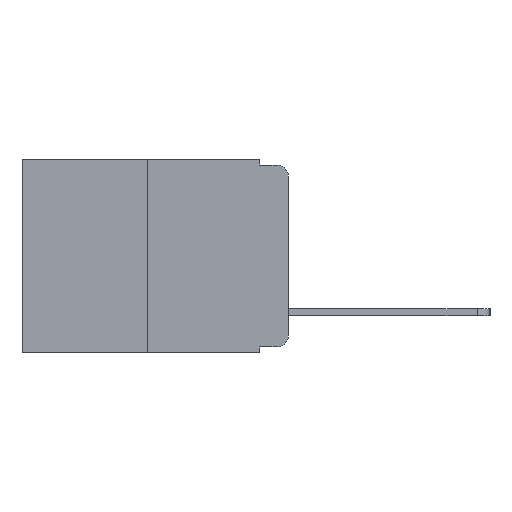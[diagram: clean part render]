
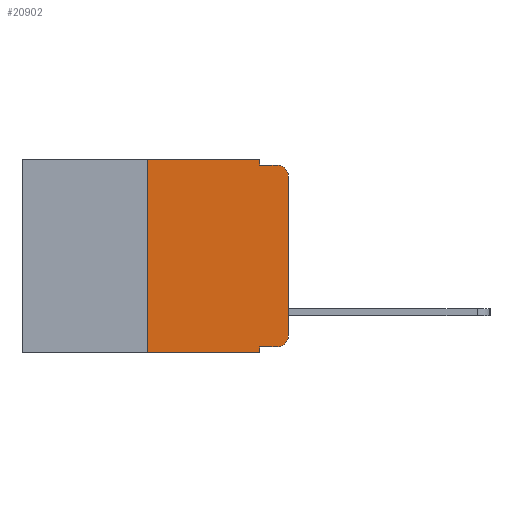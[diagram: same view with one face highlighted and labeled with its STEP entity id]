
A CAD part, left-side view. The second image highlights one B-rep face of the part: STEP entity #20902.
In plain terms, the highlighted planar face has unit normal (-1, 0, 0).
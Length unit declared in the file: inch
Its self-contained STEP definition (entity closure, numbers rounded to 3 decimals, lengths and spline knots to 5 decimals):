
#699 = LINE ( 'NONE', #13658, #19922 ) ;
#744 = VERTEX_POINT ( 'NONE', #4660 ) ;
#796 = VERTEX_POINT ( 'NONE', #8427 ) ;
#1297 = CARTESIAN_POINT ( 'NONE',  ( 0., 0.051, 0. ) ) ;
#1508 = EDGE_CURVE ( 'NONE', #4152, #19162, #22091, .T. ) ;
#1558 = VECTOR ( 'NONE', #15631, 39.37008 ) ;
#2133 = AXIS2_PLACEMENT_3D ( 'NONE', #5013, #8750, #21598 ) ;
#2367 = DIRECTION ( 'NONE',  ( 0., 0., -1. ) ) ;
#3001 = CARTESIAN_POINT ( 'NONE',  ( 0., 0.02, -0.333 ) ) ;
#3429 = LINE ( 'NONE', #10858, #8440 ) ;
#4091 = CARTESIAN_POINT ( 'NONE',  ( 0., 0., -0.313 ) ) ;
#4152 = VERTEX_POINT ( 'NONE', #13765 ) ;
#4660 = CARTESIAN_POINT ( 'NONE',  ( 0., 0.051, 0. ) ) ;
#4999 = EDGE_CURVE ( 'NONE', #8208, #7666, #699, .T. ) ;
#5013 = CARTESIAN_POINT ( 'NONE',  ( 0., 0.473, 0. ) ) ;
#5275 = DIRECTION ( 'NONE',  ( 0., -1., 0. ) ) ;
#5635 = CARTESIAN_POINT ( 'NONE',  ( 0., 0.02, -0.313 ) ) ;
#6484 = ORIENTED_EDGE ( 'NONE', *, *, #18650, .T. ) ;
#6943 = CARTESIAN_POINT ( 'NONE',  ( 0., 0.473, -0.343 ) ) ;
#7121 = VECTOR ( 'NONE', #5275, 39.37008 ) ;
#7235 = CARTESIAN_POINT ( 'NONE',  ( 0., 0., -0.03 ) ) ;
#7536 = DIRECTION ( 'NONE',  ( 0., 0., -1. ) ) ;
#7594 = ORIENTED_EDGE ( 'NONE', *, *, #1508, .F. ) ;
#7666 = VERTEX_POINT ( 'NONE', #10373 ) ;
#7857 = CARTESIAN_POINT ( 'NONE',  ( 0., 0.02, -0.03 ) ) ;
#7926 = LINE ( 'NONE', #11672, #15919 ) ;
#7987 = VERTEX_POINT ( 'NONE', #23505 ) ;
#8002 = CIRCLE ( 'NONE', #13713, 0.02 ) ;
#8208 = VERTEX_POINT ( 'NONE', #10211 ) ;
#8384 = ORIENTED_EDGE ( 'NONE', *, *, #16028, .T. ) ;
#8427 = CARTESIAN_POINT ( 'NONE',  ( 0., 0.051, -0.333 ) ) ;
#8440 = VECTOR ( 'NONE', #14536, 39.37008 ) ;
#8750 = DIRECTION ( 'NONE',  ( 1., 0., 0. ) ) ;
#9568 = EDGE_CURVE ( 'NONE', #744, #8208, #7926, .T. ) ;
#9674 = DIRECTION ( 'NONE',  ( 0., 0., -1. ) ) ;
#9736 = FACE_OUTER_BOUND ( 'NONE', #17600, .T. ) ;
#10156 = LINE ( 'NONE', #6943, #23634 ) ;
#10211 = CARTESIAN_POINT ( 'NONE',  ( 0., 0.051, -0.01 ) ) ;
#10373 = CARTESIAN_POINT ( 'NONE',  ( 0., 0.02, -0.01 ) ) ;
#10858 = CARTESIAN_POINT ( 'NONE',  ( 0., 0., 0. ) ) ;
#11388 = LINE ( 'NONE', #1297, #11942 ) ;
#11413 = CARTESIAN_POINT ( 'NONE',  ( 0., 0.25, 0. ) ) ;
#11672 = CARTESIAN_POINT ( 'NONE',  ( 0., 0.051, 0. ) ) ;
#11942 = VECTOR ( 'NONE', #18056, 39.37008 ) ;
#12091 = DIRECTION ( 'NONE',  ( 0., 0., 1. ) ) ;
#12316 = PLANE ( 'NONE',  #2133 ) ;
#13658 = CARTESIAN_POINT ( 'NONE',  ( 0., 0.051, -0.01 ) ) ;
#13713 = AXIS2_PLACEMENT_3D ( 'NONE', #7857, #20683, #9674 ) ;
#13765 = CARTESIAN_POINT ( 'NONE',  ( 0., 0.25, -0.343 ) ) ;
#13767 = CARTESIAN_POINT ( 'NONE',  ( 0., 0.473, 0. ) ) ;
#14270 = CARTESIAN_POINT ( 'NONE',  ( 0., 0.25, 0. ) ) ;
#14290 = ORIENTED_EDGE ( 'NONE', *, *, #9568, .F. ) ;
#14413 = ORIENTED_EDGE ( 'NONE', *, *, #16480, .F. ) ;
#14536 = DIRECTION ( 'NONE',  ( 0., 0., 1. ) ) ;
#14943 = DIRECTION ( 'NONE',  ( 0., -1., 0. ) ) ;
#15631 = DIRECTION ( 'NONE',  ( 0., -1., 0. ) ) ;
#15919 = VECTOR ( 'NONE', #2367, 39.37008 ) ;
#16028 = EDGE_CURVE ( 'NONE', #796, #19086, #21769, .T. ) ;
#16145 = AXIS2_PLACEMENT_3D ( 'NONE', #5635, #18503, #7536 ) ;
#16393 = LINE ( 'NONE', #13767, #1558 ) ;
#16460 = ORIENTED_EDGE ( 'NONE', *, *, #19522, .F. ) ;
#16480 = EDGE_CURVE ( 'NONE', #796, #7987, #11388, .T. ) ;
#17556 = VERTEX_POINT ( 'NONE', #4091 ) ;
#17600 = EDGE_LOOP ( 'NONE', ( #6484, #23933, #20754, #14290, #16460, #7594, #23047, #14413, #8384, #17715 ) ) ;
#17715 = ORIENTED_EDGE ( 'NONE', *, *, #21749, .T. ) ;
#17930 = DIRECTION ( 'NONE',  ( 0., -1., 0. ) ) ;
#18056 = DIRECTION ( 'NONE',  ( 0., 0., -1. ) ) ;
#18073 = CARTESIAN_POINT ( 'NONE',  ( 0., 0.051, -0.333 ) ) ;
#18503 = DIRECTION ( 'NONE',  ( -1., 0., 0. ) ) ;
#18542 = EDGE_CURVE ( 'NONE', #4152, #7987, #10156, .T. ) ;
#18650 = EDGE_CURVE ( 'NONE', #17556, #21034, #3429, .T. ) ;
#19086 = VERTEX_POINT ( 'NONE', #3001 ) ;
#19162 = VERTEX_POINT ( 'NONE', #14270 ) ;
#19522 = EDGE_CURVE ( 'NONE', #19162, #744, #16393, .T. ) ;
#19843 = CIRCLE ( 'NONE', #16145, 0.02 ) ;
#19922 = VECTOR ( 'NONE', #14943, 39.37008 ) ;
#20683 = DIRECTION ( 'NONE',  ( -1., 0., 0. ) ) ;
#20754 = ORIENTED_EDGE ( 'NONE', *, *, #4999, .F. ) ;
#20902 = ADVANCED_FACE ( 'NONE', ( #9736 ), #12316, .F. ) ;
#21034 = VERTEX_POINT ( 'NONE', #7235 ) ;
#21521 = VECTOR ( 'NONE', #12091, 39.37008 ) ;
#21598 = DIRECTION ( 'NONE',  ( 0., 0., -1. ) ) ;
#21749 = EDGE_CURVE ( 'NONE', #19086, #17556, #19843, .T. ) ;
#21769 = LINE ( 'NONE', #18073, #7121 ) ;
#22091 = LINE ( 'NONE', #11413, #21521 ) ;
#23047 = ORIENTED_EDGE ( 'NONE', *, *, #18542, .T. ) ;
#23505 = CARTESIAN_POINT ( 'NONE',  ( 0., 0.051, -0.343 ) ) ;
#23634 = VECTOR ( 'NONE', #17930, 39.37008 ) ;
#23933 = ORIENTED_EDGE ( 'NONE', *, *, #23968, .T. ) ;
#23968 = EDGE_CURVE ( 'NONE', #21034, #7666, #8002, .T. ) ;
